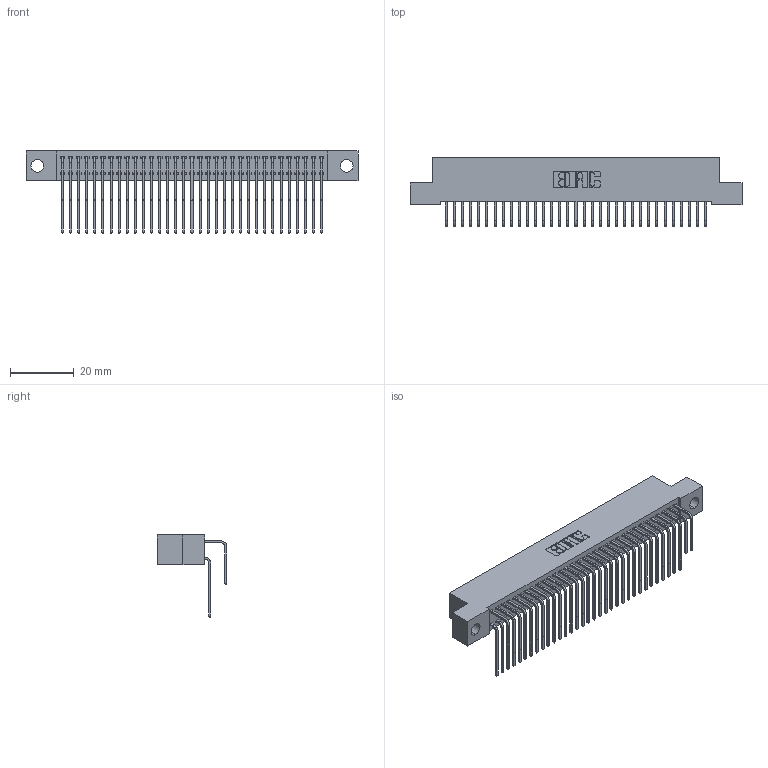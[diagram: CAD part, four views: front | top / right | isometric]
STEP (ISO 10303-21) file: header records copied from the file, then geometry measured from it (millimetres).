
FILE_DESCRIPTION (( 'STEP AP203' ), '1' );
FILE_NAME ('392-066-558-204.STEP', '2019-10-09T11:23:39', ( '' ), ( '' ), 'SwSTEP 2.0', 'SolidWorks 2016', '' );
FILE_SCHEMA (( 'CONFIG_CONTROL_DESIGN' ));
Length unit declared in the file: inch
Products named in the file (4): 342 Part_.156 TH; 345-292-001_558 559 Tail - 1; 345-292-001_558 Tail - 2; 392-066-558-204
Assembly tree (67 placements, depth 2):
  392-066-558-204
    342 Part_.156 TH
    345-292-001_558 559 Tail - 1  x33
    345-292-001_558 Tail - 2  x33
Bounding box: 104.14 x 21.91 x 25.78 mm (x, y, z)
Volume: 9608.1 mm3; surface area: 16964.3 mm2
Topology: 67 solids, 67 shells, 3674 faces, 10925 edges, 7194 vertices
Faces by surface type: plane 2574, cylinder 1100
Entity records: 24049 total; most frequent: CARTESIAN_POINT 4045, ORIENTED_EDGE 3930, DIRECTION 3453, EDGE_CURVE 1965, VECTOR 1797, LINE 1797, VERTEX_POINT 1306, AXIS2_PLACEMENT_3D 828
